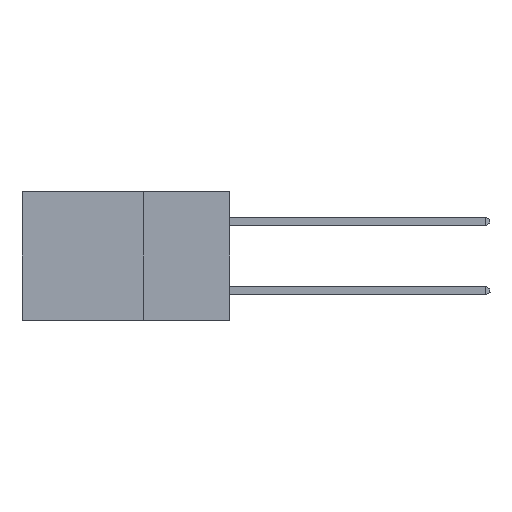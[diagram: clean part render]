
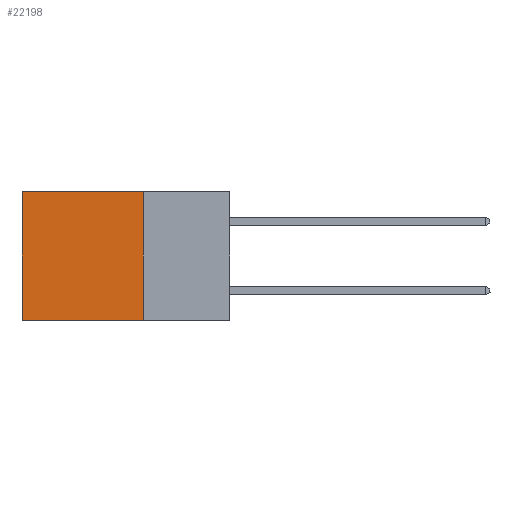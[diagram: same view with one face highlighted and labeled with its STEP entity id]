
A CAD part, left-side view. The second image highlights one B-rep face of the part: STEP entity #22198.
In plain terms, the highlighted planar face has unit normal (-1, 0, 0).
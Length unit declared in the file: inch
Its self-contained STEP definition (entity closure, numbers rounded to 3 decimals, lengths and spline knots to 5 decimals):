
#4 = VECTOR ( 'NONE', #24646, 39.37008 ) ;
#1181 = VECTOR ( 'NONE', #25347, 39.37008 ) ;
#1241 = CARTESIAN_POINT ( 'NONE',  ( 0.298, 0.25, 0. ) ) ;
#1702 = EDGE_LOOP ( 'NONE', ( #18555, #19921, #19599, #4697 ) ) ;
#3991 = VERTEX_POINT ( 'NONE', #29774 ) ;
#4697 = ORIENTED_EDGE ( 'NONE', *, *, #24401, .T. ) ;
#4975 = CARTESIAN_POINT ( 'NONE',  ( 0.298, 0.6, 0. ) ) ;
#5056 = AXIS2_PLACEMENT_3D ( 'NONE', #5254, #7918, #25217 ) ;
#5254 = CARTESIAN_POINT ( 'NONE',  ( 0.298, 0.25, 0. ) ) ;
#5679 = LINE ( 'NONE', #4975, #30365 ) ;
#7918 = DIRECTION ( 'NONE',  ( 1., 0., 0. ) ) ;
#10967 = VECTOR ( 'NONE', #23642, 39.37008 ) ;
#13876 = VERTEX_POINT ( 'NONE', #28518 ) ;
#14170 = CARTESIAN_POINT ( 'NONE',  ( 0.298, 0.6, -0.37 ) ) ;
#14863 = EDGE_CURVE ( 'NONE', #20461, #13876, #26450, .T. ) ;
#18510 = FACE_OUTER_BOUND ( 'NONE', #1702, .T. ) ;
#18555 = ORIENTED_EDGE ( 'NONE', *, *, #18670, .T. ) ;
#18670 = EDGE_CURVE ( 'NONE', #3991, #23242, #5679, .T. ) ;
#19599 = ORIENTED_EDGE ( 'NONE', *, *, #14863, .F. ) ;
#19921 = ORIENTED_EDGE ( 'NONE', *, *, #23669, .F. ) ;
#20461 = VERTEX_POINT ( 'NONE', #30277 ) ;
#22198 = ADVANCED_FACE ( 'NONE', ( #18510 ), #22769, .F. ) ;
#22769 = PLANE ( 'NONE',  #5056 ) ;
#22920 = CARTESIAN_POINT ( 'NONE',  ( 0.298, 0.25, -0.37 ) ) ;
#23242 = VERTEX_POINT ( 'NONE', #14170 ) ;
#23642 = DIRECTION ( 'NONE',  ( 0., 1., 0. ) ) ;
#23669 = EDGE_CURVE ( 'NONE', #13876, #23242, #27539, .T. ) ;
#24401 = EDGE_CURVE ( 'NONE', #20461, #3991, #30491, .T. ) ;
#24646 = DIRECTION ( 'NONE',  ( 0., 0., -1. ) ) ;
#25217 = DIRECTION ( 'NONE',  ( 0., 0., -1. ) ) ;
#25347 = DIRECTION ( 'NONE',  ( 0., 1., 0. ) ) ;
#26450 = LINE ( 'NONE', #31796, #4 ) ;
#27388 = DIRECTION ( 'NONE',  ( 0., 0., -1. ) ) ;
#27539 = LINE ( 'NONE', #22920, #1181 ) ;
#28518 = CARTESIAN_POINT ( 'NONE',  ( 0.298, 0.25, -0.37 ) ) ;
#29774 = CARTESIAN_POINT ( 'NONE',  ( 0.298, 0.6, 0. ) ) ;
#30277 = CARTESIAN_POINT ( 'NONE',  ( 0.298, 0.25, 0. ) ) ;
#30365 = VECTOR ( 'NONE', #27388, 39.37008 ) ;
#30491 = LINE ( 'NONE', #1241, #10967 ) ;
#31796 = CARTESIAN_POINT ( 'NONE',  ( 0.298, 0.25, 0. ) ) ;
